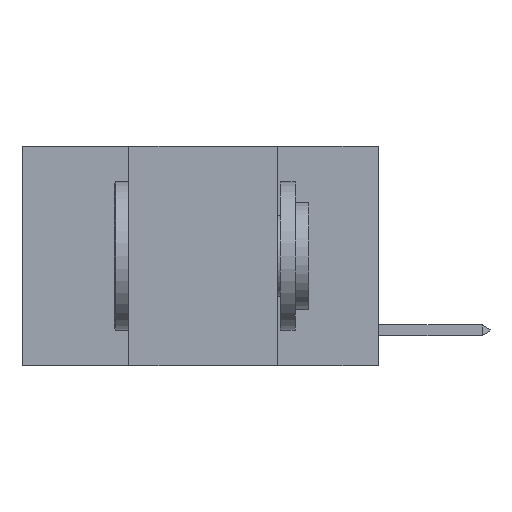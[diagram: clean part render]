
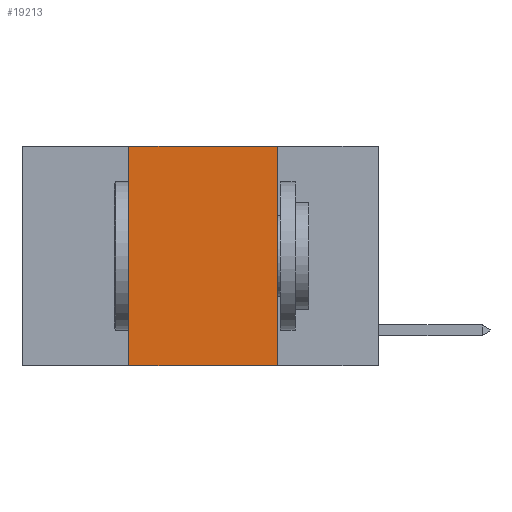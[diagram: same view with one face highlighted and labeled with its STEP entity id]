
A CAD part, left-side view. The second image highlights one B-rep face of the part: STEP entity #19213.
In plain terms, the highlighted planar face has unit normal (-1, 0, 0).
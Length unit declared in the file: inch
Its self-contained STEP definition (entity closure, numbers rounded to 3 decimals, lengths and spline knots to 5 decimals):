
#128 = ORIENTED_EDGE ( 'NONE', *, *, #17920, .T. ) ;
#351 = LINE ( 'NONE', #4160, #13307 ) ;
#633 = VECTOR ( 'NONE', #1868, 39.37008 ) ;
#714 = LINE ( 'NONE', #10581, #4297 ) ;
#1729 = EDGE_LOOP ( 'NONE', ( #2608, #19854, #16193, #128 ) ) ;
#1868 = DIRECTION ( 'NONE',  ( 0., 0., 1. ) ) ;
#2608 = ORIENTED_EDGE ( 'NONE', *, *, #17757, .F. ) ;
#3652 = EDGE_CURVE ( 'NONE', #20149, #14544, #714, .T. ) ;
#4160 = CARTESIAN_POINT ( 'NONE',  ( 0., 0.6, -0.37 ) ) ;
#4297 = VECTOR ( 'NONE', #10380, 39.37008 ) ;
#4491 = DIRECTION ( 'NONE',  ( 0., 0., -1. ) ) ;
#5732 = LINE ( 'NONE', #6825, #633 ) ;
#6825 = CARTESIAN_POINT ( 'NONE',  ( 0., 0.42, 0. ) ) ;
#7602 = CARTESIAN_POINT ( 'NONE',  ( 0., 0.6, 0. ) ) ;
#9293 = FACE_OUTER_BOUND ( 'NONE', #1729, .T. ) ;
#9402 = CARTESIAN_POINT ( 'NONE',  ( 0., 0.17, -0.37 ) ) ;
#9443 = CARTESIAN_POINT ( 'NONE',  ( 0., 0.42, 0. ) ) ;
#10380 = DIRECTION ( 'NONE',  ( 0., -1., 0. ) ) ;
#10581 = CARTESIAN_POINT ( 'NONE',  ( 0., 0.6, 0. ) ) ;
#11793 = VERTEX_POINT ( 'NONE', #15279 ) ;
#12983 = CARTESIAN_POINT ( 'NONE',  ( 0., 0.17, 0. ) ) ;
#13307 = VECTOR ( 'NONE', #15083, 39.37008 ) ;
#13865 = DIRECTION ( 'NONE',  ( 1., 0., 0. ) ) ;
#14499 = VECTOR ( 'NONE', #14505, 39.37008 ) ;
#14505 = DIRECTION ( 'NONE',  ( 0., 0., -1. ) ) ;
#14544 = VERTEX_POINT ( 'NONE', #15810 ) ;
#14965 = LINE ( 'NONE', #12983, #14499 ) ;
#15083 = DIRECTION ( 'NONE',  ( 0., -1., 0. ) ) ;
#15279 = CARTESIAN_POINT ( 'NONE',  ( 0., 0.42, -0.37 ) ) ;
#15810 = CARTESIAN_POINT ( 'NONE',  ( 0., 0.17, 0. ) ) ;
#16193 = ORIENTED_EDGE ( 'NONE', *, *, #17792, .F. ) ;
#17757 = EDGE_CURVE ( 'NONE', #14544, #19385, #14965, .T. ) ;
#17792 = EDGE_CURVE ( 'NONE', #11793, #20149, #5732, .T. ) ;
#17920 = EDGE_CURVE ( 'NONE', #11793, #19385, #351, .T. ) ;
#18458 = PLANE ( 'NONE',  #20466 ) ;
#19213 = ADVANCED_FACE ( 'NONE', ( #9293 ), #18458, .F. ) ;
#19385 = VERTEX_POINT ( 'NONE', #9402 ) ;
#19854 = ORIENTED_EDGE ( 'NONE', *, *, #3652, .F. ) ;
#20149 = VERTEX_POINT ( 'NONE', #9443 ) ;
#20466 = AXIS2_PLACEMENT_3D ( 'NONE', #7602, #13865, #4491 ) ;
